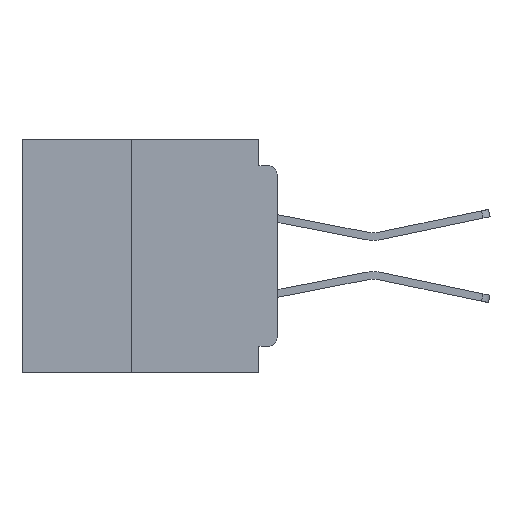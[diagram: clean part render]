
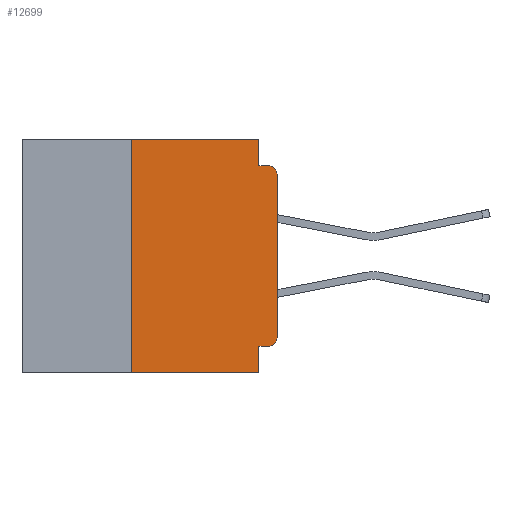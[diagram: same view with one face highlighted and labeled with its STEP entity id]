
A CAD part, left-side view. The second image highlights one B-rep face of the part: STEP entity #12699.
In plain terms, the highlighted planar face has unit normal (-1, 0, 0).
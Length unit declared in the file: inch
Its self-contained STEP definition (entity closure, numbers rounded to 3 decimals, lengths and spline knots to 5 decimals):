
#212 = VECTOR ( 'NONE', #12645, 39.37008 ) ;
#500 = CARTESIAN_POINT ( 'NONE',  ( 0., 0.015, -0.34 ) ) ;
#2865 = LINE ( 'NONE', #29053, #13740 ) ;
#3200 = DIRECTION ( 'NONE',  ( 0., 0., -1. ) ) ;
#3304 = CARTESIAN_POINT ( 'NONE',  ( 0., 0.25, -0.4 ) ) ;
#3958 = LINE ( 'NONE', #54566, #27176 ) ;
#5122 = DIRECTION ( 'NONE',  ( 0., 0., -1. ) ) ;
#5314 = CIRCLE ( 'NONE', #56590, 0.015 ) ;
#5867 = CIRCLE ( 'NONE', #26897, 0.015 ) ;
#5924 = DIRECTION ( 'NONE',  ( 0., -1., 0. ) ) ;
#6779 = CARTESIAN_POINT ( 'NONE',  ( 0., 0.437, 0. ) ) ;
#6888 = VERTEX_POINT ( 'NONE', #47305 ) ;
#6938 = VERTEX_POINT ( 'NONE', #52254 ) ;
#7019 = CARTESIAN_POINT ( 'NONE',  ( 0., 0., 0. ) ) ;
#7254 = VECTOR ( 'NONE', #11702, 39.37008 ) ;
#9521 = ORIENTED_EDGE ( 'NONE', *, *, #58384, .T. ) ;
#9759 = ORIENTED_EDGE ( 'NONE', *, *, #31609, .T. ) ;
#9761 = LINE ( 'NONE', #12207, #31456 ) ;
#9929 = EDGE_CURVE ( 'NONE', #47240, #20532, #5867, .T. ) ;
#11702 = DIRECTION ( 'NONE',  ( 0., 0., 1. ) ) ;
#12207 = CARTESIAN_POINT ( 'NONE',  ( 0., 0.437, -0.4 ) ) ;
#12645 = DIRECTION ( 'NONE',  ( 0., 1., 0. ) ) ;
#12699 = ADVANCED_FACE ( 'NONE', ( #45915 ), #39136, .F. ) ;
#12812 = CARTESIAN_POINT ( 'NONE',  ( 0., 0.031, 0. ) ) ;
#13457 = EDGE_CURVE ( 'NONE', #28991, #52654, #3958, .T. ) ;
#13740 = VECTOR ( 'NONE', #5924, 39.37008 ) ;
#13946 = EDGE_LOOP ( 'NONE', ( #9521, #54641, #32727, #23512, #51929, #24017, #33066, #44427, #26999, #9759 ) ) ;
#13972 = CARTESIAN_POINT ( 'NONE',  ( 0., 0.031, -0.045 ) ) ;
#15838 = CARTESIAN_POINT ( 'NONE',  ( 0., 0.031, -0.4 ) ) ;
#16493 = CARTESIAN_POINT ( 'NONE',  ( 0., 0., -0.045 ) ) ;
#17595 = VERTEX_POINT ( 'NONE', #15838 ) ;
#17841 = DIRECTION ( 'NONE',  ( 0., 0., -1. ) ) ;
#18479 = LINE ( 'NONE', #3304, #41550 ) ;
#18638 = LINE ( 'NONE', #23760, #32371 ) ;
#19613 = LINE ( 'NONE', #7019, #7254 ) ;
#19681 = EDGE_CURVE ( 'NONE', #20294, #6888, #18479, .T. ) ;
#20294 = VERTEX_POINT ( 'NONE', #35572 ) ;
#20532 = VERTEX_POINT ( 'NONE', #38011 ) ;
#20949 = CARTESIAN_POINT ( 'NONE',  ( 0., 0.031, -0.355 ) ) ;
#23394 = LINE ( 'NONE', #35659, #212 ) ;
#23512 = ORIENTED_EDGE ( 'NONE', *, *, #13457, .F. ) ;
#23760 = CARTESIAN_POINT ( 'NONE',  ( 0., 0.031, -0.4 ) ) ;
#24017 = ORIENTED_EDGE ( 'NONE', *, *, #19681, .F. ) ;
#25459 = DIRECTION ( 'NONE',  ( 0., 0., -1. ) ) ;
#25894 = EDGE_CURVE ( 'NONE', #20294, #17595, #9761, .T. ) ;
#26897 = AXIS2_PLACEMENT_3D ( 'NONE', #58306, #30967, #3200 ) ;
#26999 = ORIENTED_EDGE ( 'NONE', *, *, #57250, .F. ) ;
#27176 = VECTOR ( 'NONE', #17841, 39.37008 ) ;
#28991 = VERTEX_POINT ( 'NONE', #12812 ) ;
#29053 = CARTESIAN_POINT ( 'NONE',  ( 0., 0.437, 0. ) ) ;
#30967 = DIRECTION ( 'NONE',  ( -1., 0., 0. ) ) ;
#31403 = VERTEX_POINT ( 'NONE', #20949 ) ;
#31456 = VECTOR ( 'NONE', #39873, 39.37008 ) ;
#31609 = EDGE_CURVE ( 'NONE', #44693, #6938, #5314, .T. ) ;
#32371 = VECTOR ( 'NONE', #55772, 39.37008 ) ;
#32727 = ORIENTED_EDGE ( 'NONE', *, *, #32755, .F. ) ;
#32755 = EDGE_CURVE ( 'NONE', #52654, #20532, #50529, .T. ) ;
#32826 = DIRECTION ( 'NONE',  ( -1., 0., 0. ) ) ;
#33066 = ORIENTED_EDGE ( 'NONE', *, *, #25894, .T. ) ;
#35129 = EDGE_CURVE ( 'NONE', #31403, #17595, #18638, .T. ) ;
#35226 = AXIS2_PLACEMENT_3D ( 'NONE', #6779, #52855, #25459 ) ;
#35572 = CARTESIAN_POINT ( 'NONE',  ( 0., 0.25, -0.4 ) ) ;
#35659 = CARTESIAN_POINT ( 'NONE',  ( 0., 0., -0.355 ) ) ;
#38011 = CARTESIAN_POINT ( 'NONE',  ( 0., 0.015, -0.045 ) ) ;
#38432 = VECTOR ( 'NONE', #48631, 39.37008 ) ;
#39136 = PLANE ( 'NONE',  #35226 ) ;
#39873 = DIRECTION ( 'NONE',  ( 0., -1., 0. ) ) ;
#40494 = DIRECTION ( 'NONE',  ( 0., 0., 1. ) ) ;
#40797 = CARTESIAN_POINT ( 'NONE',  ( 0., 0., -0.06 ) ) ;
#41550 = VECTOR ( 'NONE', #40494, 39.37008 ) ;
#44427 = ORIENTED_EDGE ( 'NONE', *, *, #35129, .F. ) ;
#44693 = VERTEX_POINT ( 'NONE', #46800 ) ;
#45915 = FACE_OUTER_BOUND ( 'NONE', #13946, .T. ) ;
#46800 = CARTESIAN_POINT ( 'NONE',  ( 0., 0.015, -0.355 ) ) ;
#47240 = VERTEX_POINT ( 'NONE', #40797 ) ;
#47305 = CARTESIAN_POINT ( 'NONE',  ( 0., 0.25, 0. ) ) ;
#48631 = DIRECTION ( 'NONE',  ( 0., -1., 0. ) ) ;
#50529 = LINE ( 'NONE', #16493, #38432 ) ;
#51929 = ORIENTED_EDGE ( 'NONE', *, *, #58963, .F. ) ;
#52254 = CARTESIAN_POINT ( 'NONE',  ( 0., 0., -0.34 ) ) ;
#52654 = VERTEX_POINT ( 'NONE', #13972 ) ;
#52855 = DIRECTION ( 'NONE',  ( 1., 0., 0. ) ) ;
#54566 = CARTESIAN_POINT ( 'NONE',  ( 0., 0.031, 0. ) ) ;
#54641 = ORIENTED_EDGE ( 'NONE', *, *, #9929, .T. ) ;
#55772 = DIRECTION ( 'NONE',  ( 0., 0., -1. ) ) ;
#56590 = AXIS2_PLACEMENT_3D ( 'NONE', #500, #32826, #5122 ) ;
#57250 = EDGE_CURVE ( 'NONE', #44693, #31403, #23394, .T. ) ;
#58306 = CARTESIAN_POINT ( 'NONE',  ( 0., 0.015, -0.06 ) ) ;
#58384 = EDGE_CURVE ( 'NONE', #6938, #47240, #19613, .T. ) ;
#58963 = EDGE_CURVE ( 'NONE', #6888, #28991, #2865, .T. ) ;
